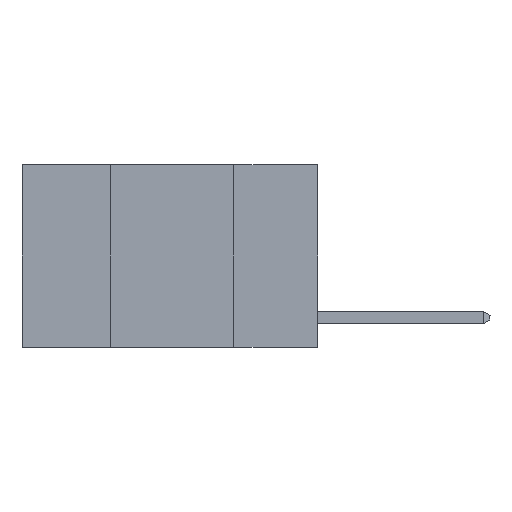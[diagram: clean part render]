
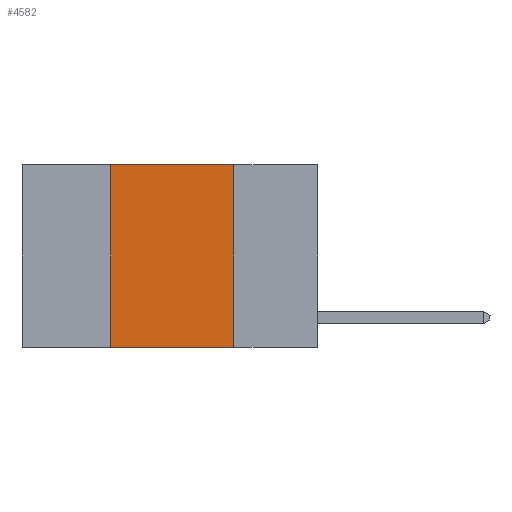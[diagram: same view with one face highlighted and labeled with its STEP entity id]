
A CAD part, left-side view. The second image highlights one B-rep face of the part: STEP entity #4582.
In plain terms, the highlighted planar face has unit normal (-1, 0, 0).
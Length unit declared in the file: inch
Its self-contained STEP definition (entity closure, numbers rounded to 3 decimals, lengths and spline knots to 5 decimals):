
#459 = CARTESIAN_POINT ( 'NONE',  ( 0., 0.17, 0. ) ) ;
#468 = CARTESIAN_POINT ( 'NONE',  ( 0., 0.42, -0.37 ) ) ;
#2905 = ORIENTED_EDGE ( 'NONE', *, *, #5124, .F. ) ;
#4329 = EDGE_LOOP ( 'NONE', ( #17206, #7398, #2905, #11527 ) ) ;
#4339 = LINE ( 'NONE', #13541, #8388 ) ;
#4582 = ADVANCED_FACE ( 'NONE', ( #5667 ), #13126, .F. ) ;
#4583 = CARTESIAN_POINT ( 'NONE',  ( 0., 0.17, 0. ) ) ;
#5124 = EDGE_CURVE ( 'NONE', #20188, #8071, #4339, .T. ) ;
#5667 = FACE_OUTER_BOUND ( 'NONE', #4329, .T. ) ;
#7087 = CARTESIAN_POINT ( 'NONE',  ( 0., 0.6, 0. ) ) ;
#7373 = CARTESIAN_POINT ( 'NONE',  ( 0., 0.6, -0.37 ) ) ;
#7398 = ORIENTED_EDGE ( 'NONE', *, *, #20649, .F. ) ;
#7822 = VERTEX_POINT ( 'NONE', #17334 ) ;
#8071 = VERTEX_POINT ( 'NONE', #13380 ) ;
#8388 = VECTOR ( 'NONE', #18027, 39.37008 ) ;
#8594 = LINE ( 'NONE', #4583, #15195 ) ;
#9006 = LINE ( 'NONE', #7087, #12515 ) ;
#11527 = ORIENTED_EDGE ( 'NONE', *, *, #19046, .T. ) ;
#11562 = EDGE_CURVE ( 'NONE', #14934, #7822, #8594, .T. ) ;
#11994 = DIRECTION ( 'NONE',  ( 0., 0., -1. ) ) ;
#12046 = DIRECTION ( 'NONE',  ( 0., 0., -1. ) ) ;
#12329 = DIRECTION ( 'NONE',  ( 0., -1., 0. ) ) ;
#12515 = VECTOR ( 'NONE', #12329, 39.37008 ) ;
#13126 = PLANE ( 'NONE',  #17823 ) ;
#13380 = CARTESIAN_POINT ( 'NONE',  ( 0., 0.42, 0. ) ) ;
#13541 = CARTESIAN_POINT ( 'NONE',  ( 0., 0.42, 0. ) ) ;
#14934 = VERTEX_POINT ( 'NONE', #459 ) ;
#15195 = VECTOR ( 'NONE', #12046, 39.37008 ) ;
#17063 = DIRECTION ( 'NONE',  ( 0., -1., 0. ) ) ;
#17206 = ORIENTED_EDGE ( 'NONE', *, *, #11562, .F. ) ;
#17334 = CARTESIAN_POINT ( 'NONE',  ( 0., 0.17, -0.37 ) ) ;
#17823 = AXIS2_PLACEMENT_3D ( 'NONE', #20591, #17869, #11994 ) ;
#17869 = DIRECTION ( 'NONE',  ( 1., 0., 0. ) ) ;
#18027 = DIRECTION ( 'NONE',  ( 0., 0., 1. ) ) ;
#18634 = LINE ( 'NONE', #7373, #18728 ) ;
#18728 = VECTOR ( 'NONE', #17063, 39.37008 ) ;
#19046 = EDGE_CURVE ( 'NONE', #20188, #7822, #18634, .T. ) ;
#20188 = VERTEX_POINT ( 'NONE', #468 ) ;
#20591 = CARTESIAN_POINT ( 'NONE',  ( 0., 0.6, 0. ) ) ;
#20649 = EDGE_CURVE ( 'NONE', #8071, #14934, #9006, .T. ) ;
